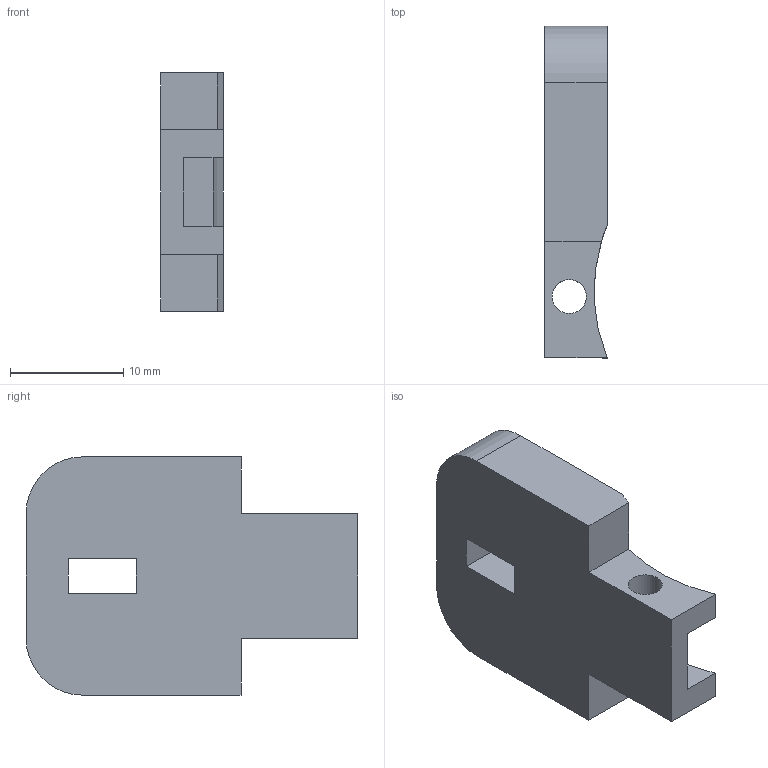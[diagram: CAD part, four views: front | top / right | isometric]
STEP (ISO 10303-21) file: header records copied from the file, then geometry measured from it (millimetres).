
FILE_DESCRIPTION((''),'2;1');
FILE_NAME('cover.stp','2013-07-01T18:25:02',('mrfr'),(''),'Autodesk Inventor 2013','Autodesk Inventor 2013','');
FILE_SCHEMA(('AUTOMOTIVE_DESIGN { 1 0 10303 214 1 1 1 1 }'));
Length unit declared in the file: millimetre
Products named in the file (1): derringer_zaver
Bounding box: 5.49 x 29.24 x 21 mm (x, y, z)
Volume: 2325.2 mm3; surface area: 1681.6 mm2
Topology: 1 solids, 1 shells, 26 faces, 72 edges, 48 vertices
Faces by surface type: plane 21, cylinder 5
Full cylindrical faces by diameter (mm): 3 x1
Entity records: 859 total; most frequent: CARTESIAN_POINT 146, ORIENTED_EDGE 142, DIRECTION 139, EDGE_CURVE 71, VECTOR 57, LINE 57, VERTEX_POINT 48, AXIS2_PLACEMENT_3D 41
